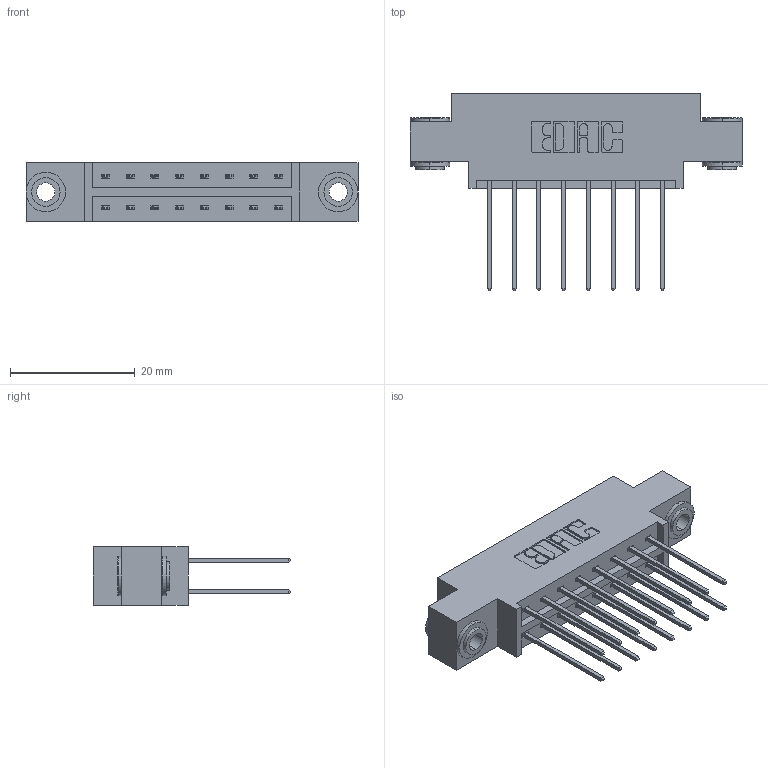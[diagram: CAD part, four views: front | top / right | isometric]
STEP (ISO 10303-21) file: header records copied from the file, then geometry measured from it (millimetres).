
FILE_DESCRIPTION (( 'STEP AP203' ), '1' );
FILE_NAME ('333-016-542-803.STEP', '2018-08-01T12:03:18', ( '' ), ( '' ), 'SwSTEP 2.0', 'SolidWorks 2016', '' );
FILE_SCHEMA (( 'CONFIG_CONTROL_DESIGN' ));
Length unit declared in the file: inch
Products named in the file (4): 345-292-001_345-293-142; 345-250-002_345-250-002-102; 333-016-542-803; 333 Part_Offset - .156 Dia - TH
Assembly tree (19 placements, depth 2):
  333-016-542-803
    333 Part_Offset - .156 Dia - TH
    345-292-001_345-293-142  x16
    345-250-002_345-250-002-102  x2
Bounding box: 53.24 x 31.63 x 9.4 mm (x, y, z)
Volume: 4983.6 mm3; surface area: 6337.2 mm2
Topology: 19 solids, 19 shells, 988 faces, 2879 edges, 1894 vertices
Faces by surface type: plane 660, cylinder 320, cone 8
Entity records: 10344 total; most frequent: CARTESIAN_POINT 1733, ORIENTED_EDGE 1662, DIRECTION 1573, EDGE_CURVE 831, VECTOR 679, LINE 679, VERTEX_POINT 550, AXIS2_PLACEMENT_3D 447
